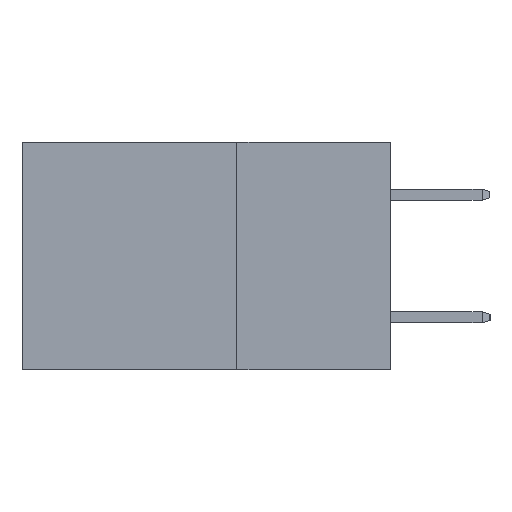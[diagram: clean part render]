
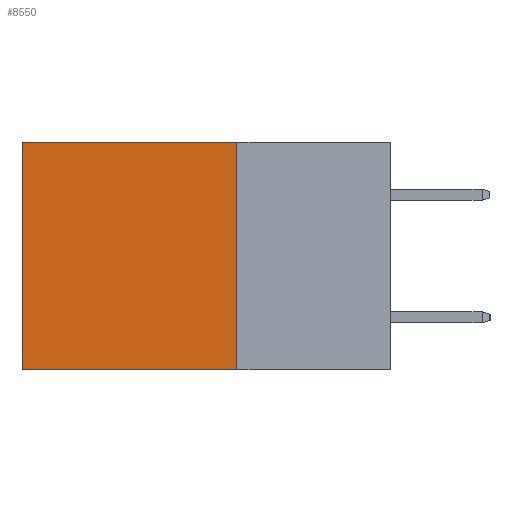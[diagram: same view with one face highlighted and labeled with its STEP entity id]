
A CAD part, left-side view. The second image highlights one B-rep face of the part: STEP entity #8550.
In plain terms, the highlighted planar face has unit normal (-1, 0, 0).
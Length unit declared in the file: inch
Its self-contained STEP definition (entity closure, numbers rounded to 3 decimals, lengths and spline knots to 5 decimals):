
#467 = CARTESIAN_POINT ( 'NONE',  ( 0.2875, 0.6, 0. ) ) ;
#728 = VECTOR ( 'NONE', #12315, 39.37008 ) ;
#3115 = CARTESIAN_POINT ( 'NONE',  ( 0.2875, 0.6, 0. ) ) ;
#3345 = CARTESIAN_POINT ( 'NONE',  ( 0.2875, 0.25, 0. ) ) ;
#4013 = CARTESIAN_POINT ( 'NONE',  ( 0.2875, 0.25, -0.37 ) ) ;
#4295 = DIRECTION ( 'NONE',  ( 0., 0., -1. ) ) ;
#4631 = VECTOR ( 'NONE', #9371, 39.37008 ) ;
#5058 = DIRECTION ( 'NONE',  ( 0., 1., 0. ) ) ;
#5315 = EDGE_CURVE ( 'NONE', #7558, #9427, #6753, .T. ) ;
#5453 = ORIENTED_EDGE ( 'NONE', *, *, #12979, .F. ) ;
#5523 = LINE ( 'NONE', #3345, #4631 ) ;
#5660 = AXIS2_PLACEMENT_3D ( 'NONE', #8871, #12121, #4295 ) ;
#6011 = LINE ( 'NONE', #12192, #12435 ) ;
#6332 = VERTEX_POINT ( 'NONE', #13949 ) ;
#6753 = LINE ( 'NONE', #3115, #728 ) ;
#7558 = VERTEX_POINT ( 'NONE', #467 ) ;
#8051 = ORIENTED_EDGE ( 'NONE', *, *, #5315, .T. ) ;
#8068 = ORIENTED_EDGE ( 'NONE', *, *, #14711, .T. ) ;
#8550 = ADVANCED_FACE ( 'NONE', ( #13313 ), #9935, .F. ) ;
#8825 = EDGE_LOOP ( 'NONE', ( #8051, #14046, #5453, #8068 ) ) ;
#8871 = CARTESIAN_POINT ( 'NONE',  ( 0.2875, 0.25, 0. ) ) ;
#9371 = DIRECTION ( 'NONE',  ( 0., 1., 0. ) ) ;
#9427 = VERTEX_POINT ( 'NONE', #12040 ) ;
#9859 = DIRECTION ( 'NONE',  ( 0., 0., -1. ) ) ;
#9935 = PLANE ( 'NONE',  #5660 ) ;
#10868 = CARTESIAN_POINT ( 'NONE',  ( 0.2875, 0.25, -0.37 ) ) ;
#11097 = VECTOR ( 'NONE', #5058, 39.37008 ) ;
#12040 = CARTESIAN_POINT ( 'NONE',  ( 0.2875, 0.6, -0.37 ) ) ;
#12121 = DIRECTION ( 'NONE',  ( 1., 0., 0. ) ) ;
#12192 = CARTESIAN_POINT ( 'NONE',  ( 0.2875, 0.25, 0. ) ) ;
#12315 = DIRECTION ( 'NONE',  ( 0., 0., -1. ) ) ;
#12435 = VECTOR ( 'NONE', #9859, 39.37008 ) ;
#12864 = LINE ( 'NONE', #10868, #11097 ) ;
#12979 = EDGE_CURVE ( 'NONE', #6332, #14343, #6011, .T. ) ;
#13313 = FACE_OUTER_BOUND ( 'NONE', #8825, .T. ) ;
#13949 = CARTESIAN_POINT ( 'NONE',  ( 0.2875, 0.25, 0. ) ) ;
#14046 = ORIENTED_EDGE ( 'NONE', *, *, #14381, .F. ) ;
#14343 = VERTEX_POINT ( 'NONE', #4013 ) ;
#14381 = EDGE_CURVE ( 'NONE', #14343, #9427, #12864, .T. ) ;
#14711 = EDGE_CURVE ( 'NONE', #6332, #7558, #5523, .T. ) ;
